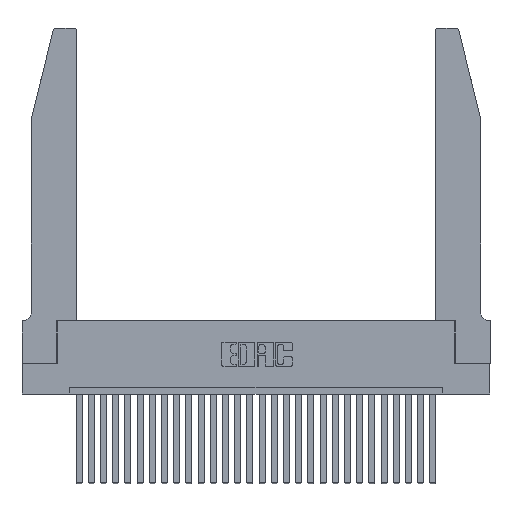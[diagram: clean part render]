
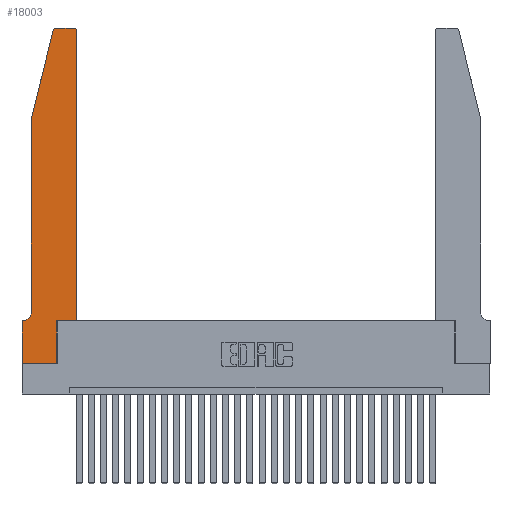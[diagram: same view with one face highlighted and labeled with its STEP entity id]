
A CAD part, top view. The second image highlights one B-rep face of the part: STEP entity #18003.
In plain terms, the highlighted planar face has unit normal (0, 0, 1).
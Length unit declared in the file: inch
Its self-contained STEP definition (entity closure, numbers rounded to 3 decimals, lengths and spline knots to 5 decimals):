
#91 = ORIENTED_EDGE ( 'NONE', *, *, #4592, .T. ) ;
#329 = VERTEX_POINT ( 'NONE', #17267 ) ;
#443 = LINE ( 'NONE', #17503, #7343 ) ;
#499 = DIRECTION ( 'NONE',  ( 1., 0., 0. ) ) ;
#593 = DIRECTION ( 'NONE',  ( 0., -1., 0. ) ) ;
#688 = DIRECTION ( 'NONE',  ( 1., 0., 0. ) ) ;
#709 = EDGE_LOOP ( 'NONE', ( #20449, #5273, #2995, #12571, #19509, #9936, #28075, #1147, #91, #7776, #4912, #23712 ) ) ;
#726 = EDGE_CURVE ( 'NONE', #7491, #986, #17848, .T. ) ;
#986 = VERTEX_POINT ( 'NONE', #1258 ) ;
#1147 = ORIENTED_EDGE ( 'NONE', *, *, #26973, .T. ) ;
#1258 = CARTESIAN_POINT ( 'NONE',  ( 0., 0.35, 0.37 ) ) ;
#1415 = EDGE_CURVE ( 'NONE', #13815, #8689, #24434, .T. ) ;
#2062 = VECTOR ( 'NONE', #2251, 39.37008 ) ;
#2160 = CARTESIAN_POINT ( 'NONE',  ( 0.4505, 0.35, 0.37 ) ) ;
#2173 = VERTEX_POINT ( 'NONE', #27191 ) ;
#2251 = DIRECTION ( 'NONE',  ( 0., 1., 0. ) ) ;
#2542 = EDGE_CURVE ( 'NONE', #28129, #12625, #9044, .T. ) ;
#2784 = DIRECTION ( 'NONE',  ( -1., 0., 0. ) ) ;
#2995 = ORIENTED_EDGE ( 'NONE', *, *, #1415, .T. ) ;
#3103 = VERTEX_POINT ( 'NONE', #28693 ) ;
#3646 = AXIS2_PLACEMENT_3D ( 'NONE', #9528, #11659, #9724 ) ;
#3651 = DIRECTION ( 'NONE',  ( 1., 0., 0. ) ) ;
#3727 = CIRCLE ( 'NONE', #24990, 0.03 ) ;
#4516 = CARTESIAN_POINT ( 'NONE',  ( 0.2865, 0.35, 0.37 ) ) ;
#4592 = EDGE_CURVE ( 'NONE', #15118, #2173, #13790, .T. ) ;
#4803 = VECTOR ( 'NONE', #499, 39.37008 ) ;
#4912 = ORIENTED_EDGE ( 'NONE', *, *, #5214, .T. ) ;
#5214 = EDGE_CURVE ( 'NONE', #19688, #3103, #18274, .T. ) ;
#5273 = ORIENTED_EDGE ( 'NONE', *, *, #8603, .T. ) ;
#7029 = CARTESIAN_POINT ( 'NONE',  ( 0., 0., 0.37 ) ) ;
#7343 = VECTOR ( 'NONE', #28617, 39.37008 ) ;
#7406 = EDGE_CURVE ( 'NONE', #986, #329, #23943, .T. ) ;
#7479 = CARTESIAN_POINT ( 'NONE',  ( 0.0755, 0.42, 0.37 ) ) ;
#7491 = VERTEX_POINT ( 'NONE', #14111 ) ;
#7776 = ORIENTED_EDGE ( 'NONE', *, *, #15401, .T. ) ;
#8165 = CARTESIAN_POINT ( 'NONE',  ( 0.2865, 0., 0.37 ) ) ;
#8557 = CARTESIAN_POINT ( 'NONE',  ( 0.284, 2.75, 0.37 ) ) ;
#8603 = EDGE_CURVE ( 'NONE', #12625, #13815, #3727, .T. ) ;
#8689 = VERTEX_POINT ( 'NONE', #24572 ) ;
#8754 = AXIS2_PLACEMENT_3D ( 'NONE', #26876, #13525, #688 ) ;
#9044 = LINE ( 'NONE', #20452, #19164 ) ;
#9528 = CARTESIAN_POINT ( 'NONE',  ( 0.0055, 0.42, 0.37 ) ) ;
#9724 = DIRECTION ( 'NONE',  ( -1., 0., 0. ) ) ;
#9936 = ORIENTED_EDGE ( 'NONE', *, *, #726, .T. ) ;
#10706 = AXIS2_PLACEMENT_3D ( 'NONE', #14691, #23846, #3651 ) ;
#11290 = CARTESIAN_POINT ( 'NONE',  ( 0.284, 2.72, 0.37 ) ) ;
#11404 = LINE ( 'NONE', #7029, #4803 ) ;
#11521 = VECTOR ( 'NONE', #13745, 39.37008 ) ;
#11659 = DIRECTION ( 'NONE',  ( 0., 0., -1. ) ) ;
#11753 = CARTESIAN_POINT ( 'NONE',  ( 0.4205, 2.75, 0.37 ) ) ;
#12299 = VECTOR ( 'NONE', #13599, 39.37008 ) ;
#12571 = ORIENTED_EDGE ( 'NONE', *, *, #15271, .T. ) ;
#12625 = VERTEX_POINT ( 'NONE', #8557 ) ;
#13525 = DIRECTION ( 'NONE',  ( 0., 0., 1. ) ) ;
#13599 = DIRECTION ( 'NONE',  ( -1., 0., 0. ) ) ;
#13745 = DIRECTION ( 'NONE',  ( 1., 0., 0. ) ) ;
#13790 = LINE ( 'NONE', #4516, #2062 ) ;
#13815 = VERTEX_POINT ( 'NONE', #17949 ) ;
#14111 = CARTESIAN_POINT ( 'NONE',  ( 0.0055, 0.35, 0.37 ) ) ;
#14691 = CARTESIAN_POINT ( 'NONE',  ( 0., 0.35, 0.37 ) ) ;
#14821 = DIRECTION ( 'NONE',  ( 1., 0., 0. ) ) ;
#15118 = VERTEX_POINT ( 'NONE', #8165 ) ;
#15271 = EDGE_CURVE ( 'NONE', #8689, #24708, #443, .T. ) ;
#15401 = EDGE_CURVE ( 'NONE', #2173, #19688, #18508, .T. ) ;
#15478 = EDGE_CURVE ( 'NONE', #3103, #28129, #18851, .T. ) ;
#17267 = CARTESIAN_POINT ( 'NONE',  ( 0., 0., 0.37 ) ) ;
#17327 = CARTESIAN_POINT ( 'NONE',  ( 0.4505, 0.35, 0.37 ) ) ;
#17503 = CARTESIAN_POINT ( 'NONE',  ( 0.0755, 2., 0.37 ) ) ;
#17848 = LINE ( 'NONE', #20720, #12299 ) ;
#17949 = CARTESIAN_POINT ( 'NONE',  ( 0.25487, 2.72718, 0.37 ) ) ;
#18003 = ADVANCED_FACE ( 'NONE', ( #24785 ), #25975, .T. ) ;
#18274 = LINE ( 'NONE', #26037, #19372 ) ;
#18508 = LINE ( 'NONE', #2160, #11521 ) ;
#18703 = DIRECTION ( 'NONE',  ( 0., 0., 1. ) ) ;
#18851 = CIRCLE ( 'NONE', #8754, 0.03 ) ;
#19164 = VECTOR ( 'NONE', #2784, 39.37008 ) ;
#19372 = VECTOR ( 'NONE', #21782, 39.37008 ) ;
#19509 = ORIENTED_EDGE ( 'NONE', *, *, #20087, .T. ) ;
#19549 = CARTESIAN_POINT ( 'NONE',  ( 0., 0., 0.37 ) ) ;
#19688 = VERTEX_POINT ( 'NONE', #17327 ) ;
#20087 = EDGE_CURVE ( 'NONE', #24708, #7491, #27099, .T. ) ;
#20449 = ORIENTED_EDGE ( 'NONE', *, *, #2542, .T. ) ;
#20452 = CARTESIAN_POINT ( 'NONE',  ( 0.2605, 2.75, 0.37 ) ) ;
#20720 = CARTESIAN_POINT ( 'NONE',  ( 0.0755, 0.35, 0.37 ) ) ;
#20826 = VECTOR ( 'NONE', #593, 39.37008 ) ;
#20962 = VECTOR ( 'NONE', #24670, 39.37008 ) ;
#21782 = DIRECTION ( 'NONE',  ( 0., 1., 0. ) ) ;
#23712 = ORIENTED_EDGE ( 'NONE', *, *, #15478, .T. ) ;
#23846 = DIRECTION ( 'NONE',  ( 0., 0., 1. ) ) ;
#23943 = LINE ( 'NONE', #19549, #20826 ) ;
#24434 = LINE ( 'NONE', #26465, #20962 ) ;
#24572 = CARTESIAN_POINT ( 'NONE',  ( 0.0755, 2., 0.37 ) ) ;
#24670 = DIRECTION ( 'NONE',  ( -0.239, -0.971, 0. ) ) ;
#24708 = VERTEX_POINT ( 'NONE', #7479 ) ;
#24785 = FACE_OUTER_BOUND ( 'NONE', #709, .T. ) ;
#24990 = AXIS2_PLACEMENT_3D ( 'NONE', #11290, #18703, #14821 ) ;
#25975 = PLANE ( 'NONE',  #10706 ) ;
#26037 = CARTESIAN_POINT ( 'NONE',  ( 0.4505, 0.35, 0.37 ) ) ;
#26465 = CARTESIAN_POINT ( 'NONE',  ( 0.0755, 2., 0.37 ) ) ;
#26876 = CARTESIAN_POINT ( 'NONE',  ( 0.4205, 2.72, 0.37 ) ) ;
#26973 = EDGE_CURVE ( 'NONE', #329, #15118, #11404, .T. ) ;
#27099 = CIRCLE ( 'NONE', #3646, 0.07 ) ;
#27191 = CARTESIAN_POINT ( 'NONE',  ( 0.2865, 0.35, 0.37 ) ) ;
#28075 = ORIENTED_EDGE ( 'NONE', *, *, #7406, .T. ) ;
#28129 = VERTEX_POINT ( 'NONE', #11753 ) ;
#28617 = DIRECTION ( 'NONE',  ( 0., -1., 0. ) ) ;
#28693 = CARTESIAN_POINT ( 'NONE',  ( 0.4505, 2.72, 0.37 ) ) ;
